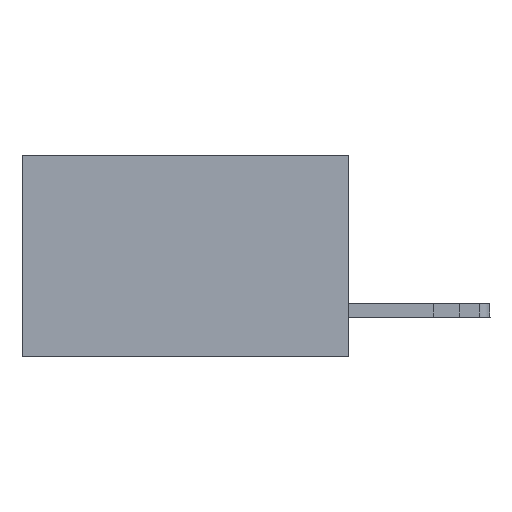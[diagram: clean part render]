
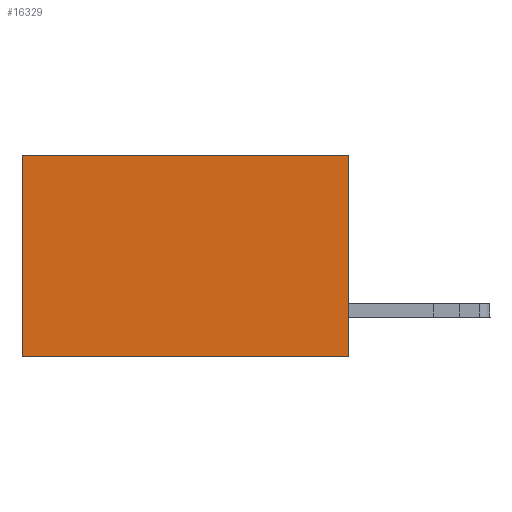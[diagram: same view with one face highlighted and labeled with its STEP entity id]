
A CAD part, left-side view. The second image highlights one B-rep face of the part: STEP entity #16329.
In plain terms, the highlighted planar face has unit normal (-1, 0, 0).
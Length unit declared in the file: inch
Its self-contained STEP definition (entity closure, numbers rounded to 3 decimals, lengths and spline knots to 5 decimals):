
#150 = DIRECTION ( 'NONE',  ( 1., 0., 0. ) ) ;
#1858 = CARTESIAN_POINT ( 'NONE',  ( 0.298, 0.6, 0. ) ) ;
#2945 = EDGE_CURVE ( 'NONE', #11315, #14664, #15020, .T. ) ;
#3345 = VERTEX_POINT ( 'NONE', #4655 ) ;
#4506 = PLANE ( 'NONE',  #15455 ) ;
#4655 = CARTESIAN_POINT ( 'NONE',  ( 0.298, 0., -0.37 ) ) ;
#4747 = VECTOR ( 'NONE', #8461, 39.37008 ) ;
#5486 = CARTESIAN_POINT ( 'NONE',  ( 0.298, 0.6, -0.37 ) ) ;
#5639 = DIRECTION ( 'NONE',  ( 0., 0., -1. ) ) ;
#8301 = EDGE_LOOP ( 'NONE', ( #12654, #13791, #23259, #14821 ) ) ;
#8461 = DIRECTION ( 'NONE',  ( 0., 0., -1. ) ) ;
#8934 = VECTOR ( 'NONE', #14377, 39.37008 ) ;
#10304 = DIRECTION ( 'NONE',  ( 0., 1., 0. ) ) ;
#10662 = LINE ( 'NONE', #25379, #8934 ) ;
#10828 = CARTESIAN_POINT ( 'NONE',  ( 0.298, 0., 0. ) ) ;
#11315 = VERTEX_POINT ( 'NONE', #12919 ) ;
#11986 = LINE ( 'NONE', #23866, #4747 ) ;
#12654 = ORIENTED_EDGE ( 'NONE', *, *, #28047, .T. ) ;
#12919 = CARTESIAN_POINT ( 'NONE',  ( 0.298, 0., 0. ) ) ;
#13438 = CARTESIAN_POINT ( 'NONE',  ( 0.298, 0., 0. ) ) ;
#13791 = ORIENTED_EDGE ( 'NONE', *, *, #17094, .F. ) ;
#14377 = DIRECTION ( 'NONE',  ( 0., 1., 0. ) ) ;
#14630 = CARTESIAN_POINT ( 'NONE',  ( 0.298, 0., 0. ) ) ;
#14664 = VERTEX_POINT ( 'NONE', #1858 ) ;
#14821 = ORIENTED_EDGE ( 'NONE', *, *, #2945, .T. ) ;
#15020 = LINE ( 'NONE', #14630, #15705 ) ;
#15455 = AXIS2_PLACEMENT_3D ( 'NONE', #13438, #150, #17731 ) ;
#15705 = VECTOR ( 'NONE', #10304, 39.37008 ) ;
#16329 = ADVANCED_FACE ( 'NONE', ( #19731 ), #4506, .F. ) ;
#17094 = EDGE_CURVE ( 'NONE', #3345, #17745, #10662, .T. ) ;
#17731 = DIRECTION ( 'NONE',  ( 0., 0., -1. ) ) ;
#17745 = VERTEX_POINT ( 'NONE', #5486 ) ;
#19731 = FACE_OUTER_BOUND ( 'NONE', #8301, .T. ) ;
#22320 = LINE ( 'NONE', #10828, #25413 ) ;
#23259 = ORIENTED_EDGE ( 'NONE', *, *, #25917, .F. ) ;
#23866 = CARTESIAN_POINT ( 'NONE',  ( 0.298, 0.6, 0. ) ) ;
#25379 = CARTESIAN_POINT ( 'NONE',  ( 0.298, 0., -0.37 ) ) ;
#25413 = VECTOR ( 'NONE', #5639, 39.37008 ) ;
#25917 = EDGE_CURVE ( 'NONE', #11315, #3345, #22320, .T. ) ;
#28047 = EDGE_CURVE ( 'NONE', #14664, #17745, #11986, .T. ) ;
